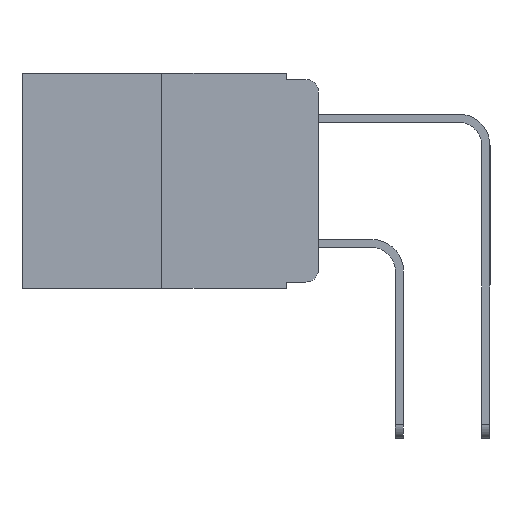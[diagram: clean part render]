
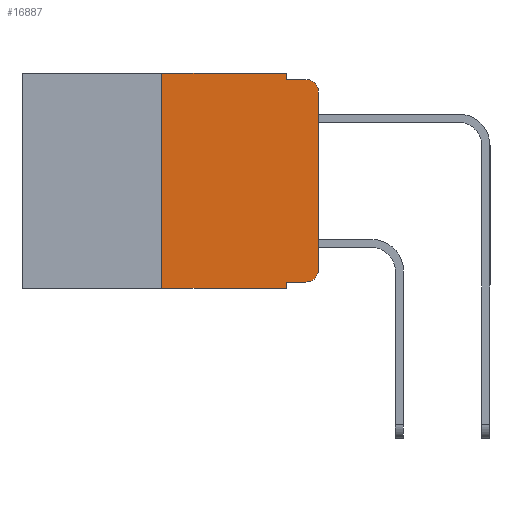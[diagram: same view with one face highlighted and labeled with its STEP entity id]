
A CAD part, left-side view. The second image highlights one B-rep face of the part: STEP entity #16887.
In plain terms, the highlighted planar face has unit normal (-1, 0, 0).
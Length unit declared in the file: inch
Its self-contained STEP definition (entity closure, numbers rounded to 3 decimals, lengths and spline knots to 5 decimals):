
#81 = CARTESIAN_POINT ( 'NONE',  ( 0., 0.051, -0.343 ) ) ;
#131 = ORIENTED_EDGE ( 'NONE', *, *, #19970, .F. ) ;
#339 = ORIENTED_EDGE ( 'NONE', *, *, #16970, .F. ) ;
#387 = ORIENTED_EDGE ( 'NONE', *, *, #544, .T. ) ;
#388 = CARTESIAN_POINT ( 'NONE',  ( 0., 0.25, -0.343 ) ) ;
#544 = EDGE_CURVE ( 'NONE', #18844, #2039, #2807, .T. ) ;
#1247 = DIRECTION ( 'NONE',  ( 0., -1., 0. ) ) ;
#1249 = ORIENTED_EDGE ( 'NONE', *, *, #3488, .F. ) ;
#1795 = EDGE_CURVE ( 'NONE', #8159, #18844, #12947, .T. ) ;
#2039 = VERTEX_POINT ( 'NONE', #18641 ) ;
#2092 = LINE ( 'NONE', #3898, #6603 ) ;
#2125 = ORIENTED_EDGE ( 'NONE', *, *, #14982, .F. ) ;
#2127 = CARTESIAN_POINT ( 'NONE',  ( 0., 0.25, 0. ) ) ;
#2379 = ORIENTED_EDGE ( 'NONE', *, *, #4038, .T. ) ;
#2512 = VERTEX_POINT ( 'NONE', #14137 ) ;
#2807 = CIRCLE ( 'NONE', #15289, 0.02 ) ;
#3068 = ORIENTED_EDGE ( 'NONE', *, *, #13999, .F. ) ;
#3488 = EDGE_CURVE ( 'NONE', #2512, #17995, #2092, .T. ) ;
#3898 = CARTESIAN_POINT ( 'NONE',  ( 0., 0.473, 0. ) ) ;
#3935 = VERTEX_POINT ( 'NONE', #12654 ) ;
#4038 = EDGE_CURVE ( 'NONE', #13422, #8476, #7896, .T. ) ;
#4105 = ORIENTED_EDGE ( 'NONE', *, *, #8868, .T. ) ;
#4861 = ORIENTED_EDGE ( 'NONE', *, *, #7833, .T. ) ;
#4967 = DIRECTION ( 'NONE',  ( 0., -1., 0. ) ) ;
#5966 = CARTESIAN_POINT ( 'NONE',  ( 0., 0.02, -0.03 ) ) ;
#6025 = CARTESIAN_POINT ( 'NONE',  ( 0., 0.02, -0.333 ) ) ;
#6338 = CARTESIAN_POINT ( 'NONE',  ( 0., 0.051, 0. ) ) ;
#6448 = ORIENTED_EDGE ( 'NONE', *, *, #1795, .T. ) ;
#6603 = VECTOR ( 'NONE', #13327, 39.37008 ) ;
#6826 = CARTESIAN_POINT ( 'NONE',  ( 0., 0.051, 0. ) ) ;
#7186 = DIRECTION ( 'NONE',  ( -1., 0., 0. ) ) ;
#7775 = CARTESIAN_POINT ( 'NONE',  ( 0., 0., -0.313 ) ) ;
#7833 = EDGE_CURVE ( 'NONE', #14435, #8159, #14021, .T. ) ;
#7896 = LINE ( 'NONE', #9747, #19011 ) ;
#7913 = VECTOR ( 'NONE', #19672, 39.37008 ) ;
#7951 = CARTESIAN_POINT ( 'NONE',  ( 0., 0.051, -0.333 ) ) ;
#8159 = VERTEX_POINT ( 'NONE', #7775 ) ;
#8375 = VECTOR ( 'NONE', #8683, 39.37008 ) ;
#8476 = VERTEX_POINT ( 'NONE', #81 ) ;
#8683 = DIRECTION ( 'NONE',  ( 0., 0., 1. ) ) ;
#8684 = VECTOR ( 'NONE', #10231, 39.37008 ) ;
#8732 = LINE ( 'NONE', #6826, #12340 ) ;
#8868 = EDGE_CURVE ( 'NONE', #10481, #14435, #19085, .T. ) ;
#9470 = FACE_OUTER_BOUND ( 'NONE', #14347, .T. ) ;
#9747 = CARTESIAN_POINT ( 'NONE',  ( 0., 0.473, -0.343 ) ) ;
#10044 = AXIS2_PLACEMENT_3D ( 'NONE', #16671, #19719, #10749 ) ;
#10201 = DIRECTION ( 'NONE',  ( -1., 0., 0. ) ) ;
#10231 = DIRECTION ( 'NONE',  ( 0., 0., 1. ) ) ;
#10481 = VERTEX_POINT ( 'NONE', #18004 ) ;
#10749 = DIRECTION ( 'NONE',  ( 0., 0., -1. ) ) ;
#11456 = DIRECTION ( 'NONE',  ( 0., 0., -1. ) ) ;
#12340 = VECTOR ( 'NONE', #11456, 39.37008 ) ;
#12654 = CARTESIAN_POINT ( 'NONE',  ( 0., 0.051, -0.01 ) ) ;
#12778 = LINE ( 'NONE', #2127, #8684 ) ;
#12947 = LINE ( 'NONE', #14744, #8375 ) ;
#13221 = DIRECTION ( 'NONE',  ( 0., 0., -1. ) ) ;
#13327 = DIRECTION ( 'NONE',  ( 0., -1., 0. ) ) ;
#13422 = VERTEX_POINT ( 'NONE', #388 ) ;
#13999 = EDGE_CURVE ( 'NONE', #10481, #8476, #8732, .T. ) ;
#14021 = CIRCLE ( 'NONE', #15528, 0.02 ) ;
#14137 = CARTESIAN_POINT ( 'NONE',  ( 0., 0.25, 0. ) ) ;
#14138 = CARTESIAN_POINT ( 'NONE',  ( 0., 0.051, 0. ) ) ;
#14347 = EDGE_LOOP ( 'NONE', ( #6448, #387, #131, #339, #1249, #2125, #2379, #3068, #4105, #4861 ) ) ;
#14435 = VERTEX_POINT ( 'NONE', #6025 ) ;
#14744 = CARTESIAN_POINT ( 'NONE',  ( 0., 0., 0. ) ) ;
#14982 = EDGE_CURVE ( 'NONE', #13422, #2512, #12778, .T. ) ;
#15118 = VECTOR ( 'NONE', #1247, 39.37008 ) ;
#15195 = CARTESIAN_POINT ( 'NONE',  ( 0., 0.051, -0.01 ) ) ;
#15289 = AXIS2_PLACEMENT_3D ( 'NONE', #5966, #10201, #13221 ) ;
#15489 = DIRECTION ( 'NONE',  ( 0., 0., -1. ) ) ;
#15528 = AXIS2_PLACEMENT_3D ( 'NONE', #16277, #7186, #17779 ) ;
#15621 = VECTOR ( 'NONE', #15489, 39.37008 ) ;
#16277 = CARTESIAN_POINT ( 'NONE',  ( 0., 0.02, -0.313 ) ) ;
#16671 = CARTESIAN_POINT ( 'NONE',  ( 0., 0.473, 0. ) ) ;
#16887 = ADVANCED_FACE ( 'NONE', ( #9470 ), #18235, .F. ) ;
#16970 = EDGE_CURVE ( 'NONE', #17995, #3935, #19122, .T. ) ;
#17302 = CARTESIAN_POINT ( 'NONE',  ( 0., 0., -0.03 ) ) ;
#17779 = DIRECTION ( 'NONE',  ( 0., 0., -1. ) ) ;
#17995 = VERTEX_POINT ( 'NONE', #14138 ) ;
#18004 = CARTESIAN_POINT ( 'NONE',  ( 0., 0.051, -0.333 ) ) ;
#18235 = PLANE ( 'NONE',  #10044 ) ;
#18641 = CARTESIAN_POINT ( 'NONE',  ( 0., 0.02, -0.01 ) ) ;
#18844 = VERTEX_POINT ( 'NONE', #17302 ) ;
#19011 = VECTOR ( 'NONE', #4967, 39.37008 ) ;
#19085 = LINE ( 'NONE', #7951, #15118 ) ;
#19122 = LINE ( 'NONE', #6338, #15621 ) ;
#19672 = DIRECTION ( 'NONE',  ( 0., -1., 0. ) ) ;
#19719 = DIRECTION ( 'NONE',  ( 1., 0., 0. ) ) ;
#19970 = EDGE_CURVE ( 'NONE', #3935, #2039, #20411, .T. ) ;
#20411 = LINE ( 'NONE', #15195, #7913 ) ;
